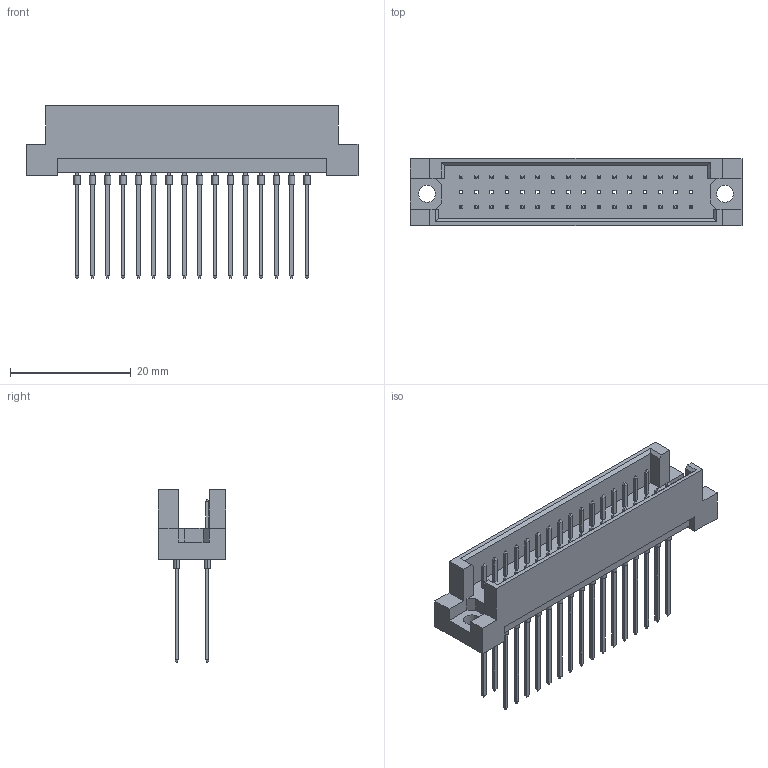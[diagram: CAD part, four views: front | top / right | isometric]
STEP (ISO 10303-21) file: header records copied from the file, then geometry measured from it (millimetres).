
FILE_DESCRIPTION (( 'STEP AP203' ), '1' );
FILE_NAME ('493-132-281-611.STEP', '2019-11-11T20:26:49', ( '' ), ( '' ), 'SwSTEP 2.0', 'SolidWorks 2020', '' );
FILE_SCHEMA (( 'CONFIG_CONTROL_DESIGN' ));
Length unit declared in the file: millimetre
Products named in the file (3): 493-290_81; 493-132-281-611; 493 Part_48
Assembly tree (33 placements, depth 2):
  493-132-281-611
    493 Part_48
    493-290_81  x32
Bounding box: 55 x 11.1 x 28.6 mm (x, y, z)
Volume: 3551.1 mm3; surface area: 5720.9 mm2
Topology: 33 solids, 33 shells, 948 faces, 2194 edges, 1376 vertices
Faces by surface type: plane 880, cylinder 68
Entity records: 10045 total; most frequent: CARTESIAN_POINT 1578, ORIENTED_EDGE 1536, DIRECTION 1384, EDGE_CURVE 768, LINE 756, VECTOR 756, VERTEX_POINT 508, EDGE_LOOP 368
